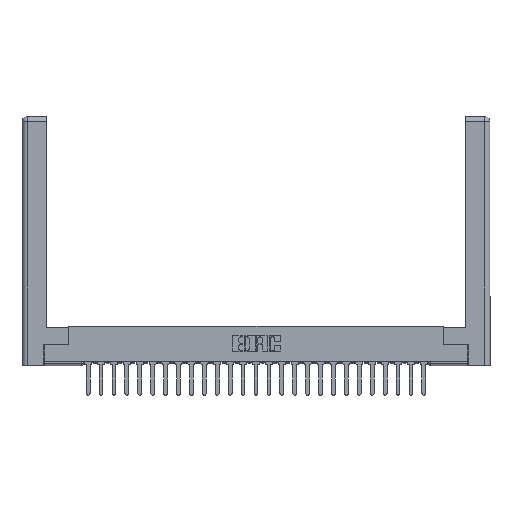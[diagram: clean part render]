
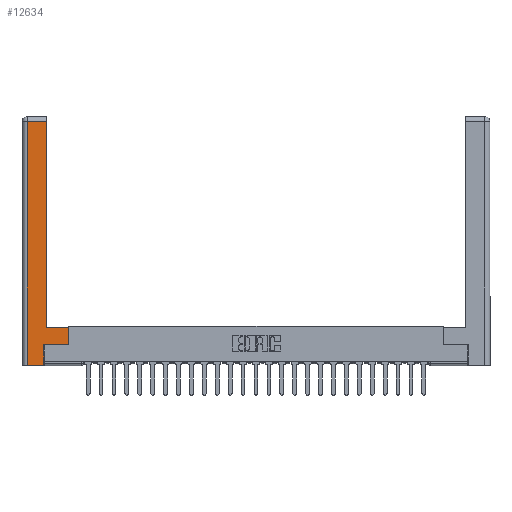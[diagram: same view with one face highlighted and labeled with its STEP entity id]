
A CAD part, top view. The second image highlights one B-rep face of the part: STEP entity #12634.
In plain terms, the highlighted planar face has unit normal (0, 0, 1).
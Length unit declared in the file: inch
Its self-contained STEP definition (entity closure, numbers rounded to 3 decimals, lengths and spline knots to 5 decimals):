
#3 = VERTEX_POINT ( 'NONE', #6528 ) ;
#375 = CARTESIAN_POINT ( 'NONE',  ( 0.265, 0., 0. ) ) ;
#527 = ORIENTED_EDGE ( 'NONE', *, *, #15348, .T. ) ;
#783 = CARTESIAN_POINT ( 'NONE',  ( 0.0615, 0., 0. ) ) ;
#889 = CARTESIAN_POINT ( 'NONE',  ( 0.0615, 2.94, 0. ) ) ;
#998 = LINE ( 'NONE', #13706, #5515 ) ;
#2320 = CARTESIAN_POINT ( 'NONE',  ( 0.0615, 0., 0. ) ) ;
#2590 = LINE ( 'NONE', #783, #18851 ) ;
#4371 = CARTESIAN_POINT ( 'NONE',  ( 0.565, 0.45, 0. ) ) ;
#4726 = VERTEX_POINT ( 'NONE', #2320 ) ;
#5515 = VECTOR ( 'NONE', #20262, 39.37008 ) ;
#5797 = EDGE_CURVE ( 'NONE', #16068, #21132, #7623, .T. ) ;
#5834 = CARTESIAN_POINT ( 'NONE',  ( 0.265, 0.245, 0. ) ) ;
#6528 = CARTESIAN_POINT ( 'NONE',  ( 0.565, 0.245, 0. ) ) ;
#6535 = DIRECTION ( 'NONE',  ( 0., 0., -1. ) ) ;
#7623 = LINE ( 'NONE', #20895, #15102 ) ;
#8316 = VECTOR ( 'NONE', #26782, 39.37008 ) ;
#8527 = CARTESIAN_POINT ( 'NONE',  ( 0.565, 0.45, 0. ) ) ;
#8708 = ORIENTED_EDGE ( 'NONE', *, *, #5797, .T. ) ;
#8731 = DIRECTION ( 'NONE',  ( 1., 0., 0. ) ) ;
#8916 = FACE_OUTER_BOUND ( 'NONE', #18691, .T. ) ;
#8938 = EDGE_CURVE ( 'NONE', #21132, #4726, #2590, .T. ) ;
#9025 = VERTEX_POINT ( 'NONE', #18354 ) ;
#9352 = CARTESIAN_POINT ( 'NONE',  ( 0.265, 0.245, 0. ) ) ;
#9382 = ORIENTED_EDGE ( 'NONE', *, *, #12108, .T. ) ;
#10140 = CARTESIAN_POINT ( 'NONE',  ( 0.295, 3., 0. ) ) ;
#10873 = CARTESIAN_POINT ( 'NONE',  ( 0.565, 0.245, 0. ) ) ;
#11778 = VECTOR ( 'NONE', #16518, 39.37008 ) ;
#11805 = AXIS2_PLACEMENT_3D ( 'NONE', #21501, #6535, #26108 ) ;
#12108 = EDGE_CURVE ( 'NONE', #3, #27125, #18887, .T. ) ;
#12355 = EDGE_CURVE ( 'NONE', #27125, #9025, #998, .T. ) ;
#12634 = ADVANCED_FACE ( 'NONE', ( #8916 ), #12841, .F. ) ;
#12699 = LINE ( 'NONE', #10873, #13163 ) ;
#12771 = ORIENTED_EDGE ( 'NONE', *, *, #26670, .T. ) ;
#12841 = PLANE ( 'NONE',  #11805 ) ;
#13163 = VECTOR ( 'NONE', #21213, 39.37008 ) ;
#13706 = CARTESIAN_POINT ( 'NONE',  ( 0.295, 0.45, 0. ) ) ;
#14367 = VECTOR ( 'NONE', #18153, 39.37008 ) ;
#15102 = VECTOR ( 'NONE', #16148, 39.37008 ) ;
#15348 = EDGE_CURVE ( 'NONE', #9025, #16068, #23143, .T. ) ;
#16068 = VERTEX_POINT ( 'NONE', #23796 ) ;
#16148 = DIRECTION ( 'NONE',  ( -1., 0., 0. ) ) ;
#16518 = DIRECTION ( 'NONE',  ( 0., 1., 0. ) ) ;
#17413 = CARTESIAN_POINT ( 'NONE',  ( 0.265, 0., 0. ) ) ;
#17610 = VECTOR ( 'NONE', #8731, 39.37008 ) ;
#18153 = DIRECTION ( 'NONE',  ( 0., 1., 0. ) ) ;
#18354 = CARTESIAN_POINT ( 'NONE',  ( 0.295, 0.45, 0. ) ) ;
#18410 = VERTEX_POINT ( 'NONE', #5834 ) ;
#18691 = EDGE_LOOP ( 'NONE', ( #527, #8708, #24032, #12771, #24169, #26593, #9382, #19847 ) ) ;
#18851 = VECTOR ( 'NONE', #21876, 39.37008 ) ;
#18887 = LINE ( 'NONE', #8527, #11778 ) ;
#19847 = ORIENTED_EDGE ( 'NONE', *, *, #12355, .T. ) ;
#20242 = LINE ( 'NONE', #9352, #14367 ) ;
#20262 = DIRECTION ( 'NONE',  ( -1., 0., 0. ) ) ;
#20538 = VERTEX_POINT ( 'NONE', #375 ) ;
#20895 = CARTESIAN_POINT ( 'NONE',  ( 0.0615, 2.94, 0. ) ) ;
#21132 = VERTEX_POINT ( 'NONE', #889 ) ;
#21213 = DIRECTION ( 'NONE',  ( 1., 0., 0. ) ) ;
#21322 = LINE ( 'NONE', #17413, #17610 ) ;
#21501 = CARTESIAN_POINT ( 'NONE',  ( 0., 0., 0. ) ) ;
#21876 = DIRECTION ( 'NONE',  ( 0., -1., 0. ) ) ;
#23012 = EDGE_CURVE ( 'NONE', #20538, #18410, #20242, .T. ) ;
#23143 = LINE ( 'NONE', #10140, #8316 ) ;
#23796 = CARTESIAN_POINT ( 'NONE',  ( 0.295, 2.94, 0. ) ) ;
#24032 = ORIENTED_EDGE ( 'NONE', *, *, #8938, .T. ) ;
#24169 = ORIENTED_EDGE ( 'NONE', *, *, #23012, .T. ) ;
#26108 = DIRECTION ( 'NONE',  ( -1., 0., 0. ) ) ;
#26593 = ORIENTED_EDGE ( 'NONE', *, *, #27580, .T. ) ;
#26670 = EDGE_CURVE ( 'NONE', #4726, #20538, #21322, .T. ) ;
#26782 = DIRECTION ( 'NONE',  ( 0., 1., 0. ) ) ;
#27125 = VERTEX_POINT ( 'NONE', #4371 ) ;
#27580 = EDGE_CURVE ( 'NONE', #18410, #3, #12699, .T. ) ;
